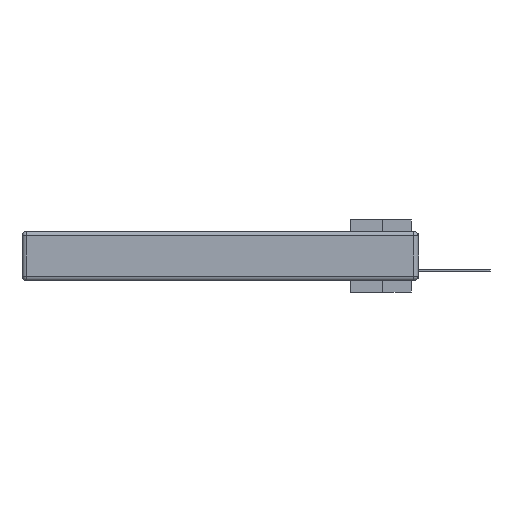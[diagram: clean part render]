
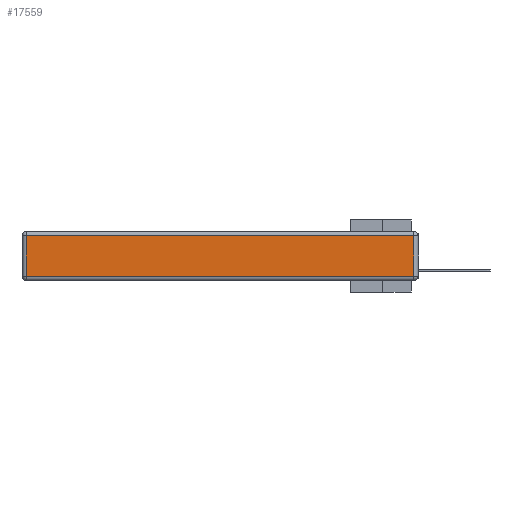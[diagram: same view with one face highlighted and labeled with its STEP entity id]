
A CAD part, left-side view. The second image highlights one B-rep face of the part: STEP entity #17559.
In plain terms, the highlighted planar face has unit normal (-1, 0, 0).
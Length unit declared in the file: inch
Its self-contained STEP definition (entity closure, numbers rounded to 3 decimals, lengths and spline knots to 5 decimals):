
#47 = VECTOR ( 'NONE', #17243, 39.37008 ) ;
#655 = CARTESIAN_POINT ( 'NONE',  ( 0., 0.03, -0.343 ) ) ;
#1095 = DIRECTION ( 'NONE',  ( 0., 0., 1. ) ) ;
#1363 = CARTESIAN_POINT ( 'NONE',  ( 0., 0., -0.313 ) ) ;
#1555 = CARTESIAN_POINT ( 'NONE',  ( 0., 2.72, -0.313 ) ) ;
#2360 = VECTOR ( 'NONE', #14689, 39.37008 ) ;
#2470 = PLANE ( 'NONE',  #3172 ) ;
#3172 = AXIS2_PLACEMENT_3D ( 'NONE', #5182, #14432, #12157 ) ;
#3441 = LINE ( 'NONE', #5870, #47 ) ;
#4454 = ORIENTED_EDGE ( 'NONE', *, *, #10634, .T. ) ;
#5182 = CARTESIAN_POINT ( 'NONE',  ( 0., 0., -0.343 ) ) ;
#5870 = CARTESIAN_POINT ( 'NONE',  ( 0., 2.72, -0.343 ) ) ;
#6364 = VERTEX_POINT ( 'NONE', #14086 ) ;
#7630 = CARTESIAN_POINT ( 'NONE',  ( 0., 0.03, -0.03 ) ) ;
#8497 = LINE ( 'NONE', #1363, #14044 ) ;
#10009 = LINE ( 'NONE', #19218, #2360 ) ;
#10615 = DIRECTION ( 'NONE',  ( 0., -1., 0. ) ) ;
#10634 = EDGE_CURVE ( 'NONE', #21604, #11998, #10009, .T. ) ;
#11998 = VERTEX_POINT ( 'NONE', #15718 ) ;
#12157 = DIRECTION ( 'NONE',  ( 0., 0., 1. ) ) ;
#13606 = ORIENTED_EDGE ( 'NONE', *, *, #22219, .T. ) ;
#14044 = VECTOR ( 'NONE', #10615, 39.37008 ) ;
#14086 = CARTESIAN_POINT ( 'NONE',  ( 0., 0.03, -0.313 ) ) ;
#14432 = DIRECTION ( 'NONE',  ( -1., 0., 0. ) ) ;
#14689 = DIRECTION ( 'NONE',  ( 0., 1., 0. ) ) ;
#15718 = CARTESIAN_POINT ( 'NONE',  ( 0., 2.72, -0.03 ) ) ;
#16313 = EDGE_LOOP ( 'NONE', ( #13606, #22900, #4454, #18949 ) ) ;
#17243 = DIRECTION ( 'NONE',  ( 0., 0., -1. ) ) ;
#17559 = ADVANCED_FACE ( 'NONE', ( #25930 ), #2470, .T. ) ;
#18949 = ORIENTED_EDGE ( 'NONE', *, *, #24414, .T. ) ;
#19218 = CARTESIAN_POINT ( 'NONE',  ( 0., 2.75, -0.03 ) ) ;
#21410 = LINE ( 'NONE', #655, #27176 ) ;
#21604 = VERTEX_POINT ( 'NONE', #7630 ) ;
#22219 = EDGE_CURVE ( 'NONE', #27975, #6364, #8497, .T. ) ;
#22900 = ORIENTED_EDGE ( 'NONE', *, *, #25354, .T. ) ;
#24414 = EDGE_CURVE ( 'NONE', #11998, #27975, #3441, .T. ) ;
#25354 = EDGE_CURVE ( 'NONE', #6364, #21604, #21410, .T. ) ;
#25930 = FACE_OUTER_BOUND ( 'NONE', #16313, .T. ) ;
#27176 = VECTOR ( 'NONE', #1095, 39.37008 ) ;
#27975 = VERTEX_POINT ( 'NONE', #1555 ) ;
